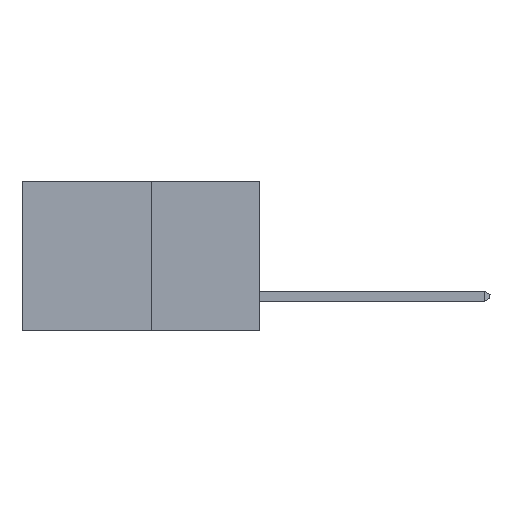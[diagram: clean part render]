
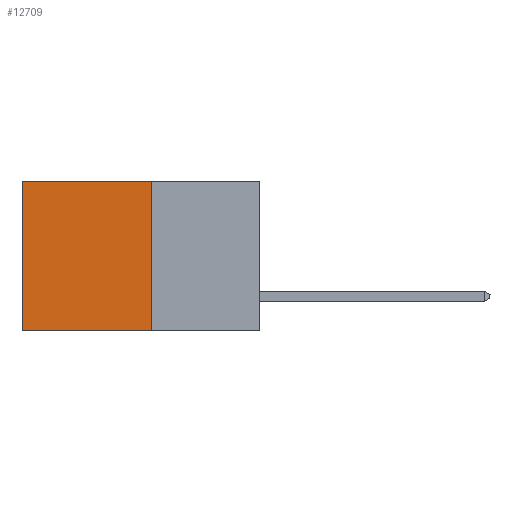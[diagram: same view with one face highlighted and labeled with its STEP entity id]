
A CAD part, left-side view. The second image highlights one B-rep face of the part: STEP entity #12709.
In plain terms, the highlighted planar face has unit normal (-1, 0, 0).
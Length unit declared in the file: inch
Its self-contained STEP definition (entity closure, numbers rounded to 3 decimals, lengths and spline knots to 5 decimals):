
#642 = CARTESIAN_POINT ( 'NONE',  ( 0.277, 0.27, -0.37 ) ) ;
#1639 = VERTEX_POINT ( 'NONE', #2350 ) ;
#1784 = VERTEX_POINT ( 'NONE', #3702 ) ;
#2350 = CARTESIAN_POINT ( 'NONE',  ( 0.277, 0.59, -0.37 ) ) ;
#3232 = ORIENTED_EDGE ( 'NONE', *, *, #20251, .F. ) ;
#3702 = CARTESIAN_POINT ( 'NONE',  ( 0.277, 0.27, 0. ) ) ;
#4227 = VECTOR ( 'NONE', #7188, 39.37008 ) ;
#4637 = EDGE_CURVE ( 'NONE', #15680, #1639, #24910, .T. ) ;
#4729 = DIRECTION ( 'NONE',  ( 1., 0., 0. ) ) ;
#4898 = CARTESIAN_POINT ( 'NONE',  ( 0.277, 0.59, 0. ) ) ;
#7050 = VECTOR ( 'NONE', #19179, 39.37008 ) ;
#7188 = DIRECTION ( 'NONE',  ( 0., 0., -1. ) ) ;
#7267 = EDGE_LOOP ( 'NONE', ( #15214, #22156, #3232, #23678 ) ) ;
#7410 = CARTESIAN_POINT ( 'NONE',  ( 0.277, 0.59, -0.37 ) ) ;
#7964 = VECTOR ( 'NONE', #24287, 39.37008 ) ;
#10514 = PLANE ( 'NONE',  #20073 ) ;
#12256 = LINE ( 'NONE', #24852, #7050 ) ;
#12709 = ADVANCED_FACE ( 'NONE', ( #15791 ), #10514, .F. ) ;
#12778 = VECTOR ( 'NONE', #14378, 39.37008 ) ;
#13842 = LINE ( 'NONE', #20464, #7964 ) ;
#14378 = DIRECTION ( 'NONE',  ( 0., 0., -1. ) ) ;
#14978 = EDGE_CURVE ( 'NONE', #17703, #1639, #13842, .T. ) ;
#15214 = ORIENTED_EDGE ( 'NONE', *, *, #4637, .T. ) ;
#15680 = VERTEX_POINT ( 'NONE', #4898 ) ;
#15791 = FACE_OUTER_BOUND ( 'NONE', #7267, .T. ) ;
#16470 = CARTESIAN_POINT ( 'NONE',  ( 0.277, 0.27, -0.37 ) ) ;
#17366 = LINE ( 'NONE', #642, #12778 ) ;
#17703 = VERTEX_POINT ( 'NONE', #20342 ) ;
#18415 = DIRECTION ( 'NONE',  ( 0., 0., -1. ) ) ;
#19179 = DIRECTION ( 'NONE',  ( 0., 1., 0. ) ) ;
#20073 = AXIS2_PLACEMENT_3D ( 'NONE', #16470, #4729, #18415 ) ;
#20251 = EDGE_CURVE ( 'NONE', #1784, #17703, #17366, .T. ) ;
#20342 = CARTESIAN_POINT ( 'NONE',  ( 0.277, 0.27, -0.37 ) ) ;
#20464 = CARTESIAN_POINT ( 'NONE',  ( 0.277, 0.27, -0.37 ) ) ;
#22156 = ORIENTED_EDGE ( 'NONE', *, *, #14978, .F. ) ;
#23678 = ORIENTED_EDGE ( 'NONE', *, *, #24503, .T. ) ;
#24287 = DIRECTION ( 'NONE',  ( 0., 1., 0. ) ) ;
#24503 = EDGE_CURVE ( 'NONE', #1784, #15680, #12256, .T. ) ;
#24852 = CARTESIAN_POINT ( 'NONE',  ( 0.277, 0.27, 0. ) ) ;
#24910 = LINE ( 'NONE', #7410, #4227 ) ;
